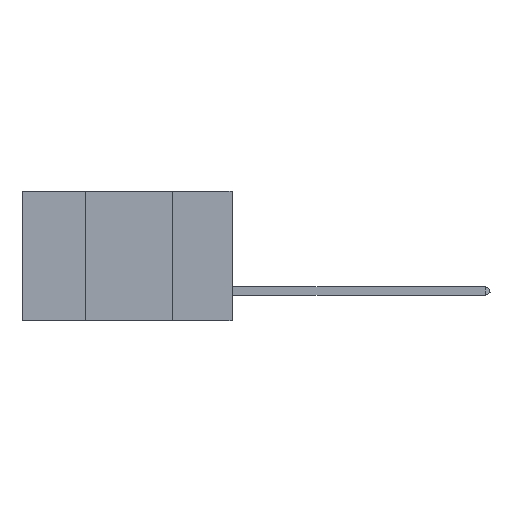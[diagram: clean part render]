
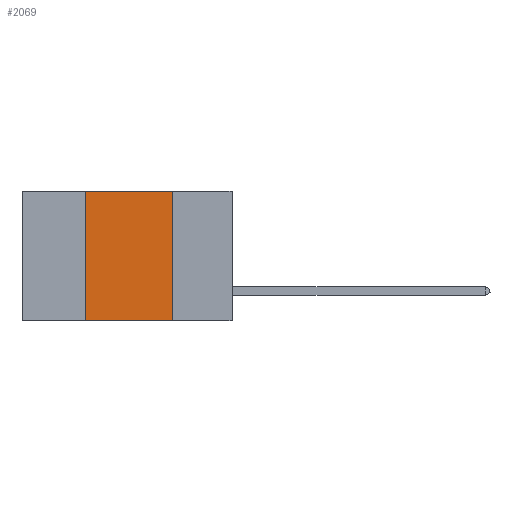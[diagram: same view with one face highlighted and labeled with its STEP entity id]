
A CAD part, left-side view. The second image highlights one B-rep face of the part: STEP entity #2069.
In plain terms, the highlighted planar face has unit normal (-1, 0, 0).
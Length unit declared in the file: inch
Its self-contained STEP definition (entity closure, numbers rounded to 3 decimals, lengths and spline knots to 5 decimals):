
#171 = LINE ( 'NONE', #4747, #10922 ) ;
#181 = LINE ( 'NONE', #15124, #5743 ) ;
#531 = ORIENTED_EDGE ( 'NONE', *, *, #770, .T. ) ;
#656 = VERTEX_POINT ( 'NONE', #24521 ) ;
#770 = EDGE_CURVE ( 'NONE', #17454, #656, #20507, .T. ) ;
#1127 = EDGE_CURVE ( 'NONE', #18845, #8250, #2653, .T. ) ;
#2069 = ADVANCED_FACE ( 'NONE', ( #15819 ), #23779, .F. ) ;
#2653 = LINE ( 'NONE', #5079, #22974 ) ;
#3452 = DIRECTION ( 'NONE',  ( 0., 0., -1. ) ) ;
#3520 = DIRECTION ( 'NONE',  ( 0., 0., 1. ) ) ;
#4747 = CARTESIAN_POINT ( 'NONE',  ( 0., 0.17, 0. ) ) ;
#4796 = VECTOR ( 'NONE', #20516, 39.37008 ) ;
#5079 = CARTESIAN_POINT ( 'NONE',  ( 0., 0.6, 0. ) ) ;
#5743 = VECTOR ( 'NONE', #3520, 39.37008 ) ;
#6408 = ORIENTED_EDGE ( 'NONE', *, *, #1127, .F. ) ;
#6894 = CARTESIAN_POINT ( 'NONE',  ( 0., 0.6, -0.37 ) ) ;
#8250 = VERTEX_POINT ( 'NONE', #25492 ) ;
#8872 = DIRECTION ( 'NONE',  ( 0., 0., -1. ) ) ;
#10664 = ORIENTED_EDGE ( 'NONE', *, *, #17397, .F. ) ;
#10922 = VECTOR ( 'NONE', #8872, 39.37008 ) ;
#14271 = AXIS2_PLACEMENT_3D ( 'NONE', #16780, #17113, #3452 ) ;
#15124 = CARTESIAN_POINT ( 'NONE',  ( 0., 0.42, 0. ) ) ;
#15819 = FACE_OUTER_BOUND ( 'NONE', #18057, .T. ) ;
#16225 = CARTESIAN_POINT ( 'NONE',  ( 0., 0.42, 0. ) ) ;
#16780 = CARTESIAN_POINT ( 'NONE',  ( 0., 0.6, 0. ) ) ;
#17113 = DIRECTION ( 'NONE',  ( 1., 0., 0. ) ) ;
#17397 = EDGE_CURVE ( 'NONE', #17454, #18845, #181, .T. ) ;
#17454 = VERTEX_POINT ( 'NONE', #22892 ) ;
#18057 = EDGE_LOOP ( 'NONE', ( #23118, #6408, #10664, #531 ) ) ;
#18845 = VERTEX_POINT ( 'NONE', #16225 ) ;
#20236 = EDGE_CURVE ( 'NONE', #8250, #656, #171, .T. ) ;
#20507 = LINE ( 'NONE', #6894, #4796 ) ;
#20516 = DIRECTION ( 'NONE',  ( 0., -1., 0. ) ) ;
#22838 = DIRECTION ( 'NONE',  ( 0., -1., 0. ) ) ;
#22892 = CARTESIAN_POINT ( 'NONE',  ( 0., 0.42, -0.37 ) ) ;
#22974 = VECTOR ( 'NONE', #22838, 39.37008 ) ;
#23118 = ORIENTED_EDGE ( 'NONE', *, *, #20236, .F. ) ;
#23779 = PLANE ( 'NONE',  #14271 ) ;
#24521 = CARTESIAN_POINT ( 'NONE',  ( 0., 0.17, -0.37 ) ) ;
#25492 = CARTESIAN_POINT ( 'NONE',  ( 0., 0.17, 0. ) ) ;
